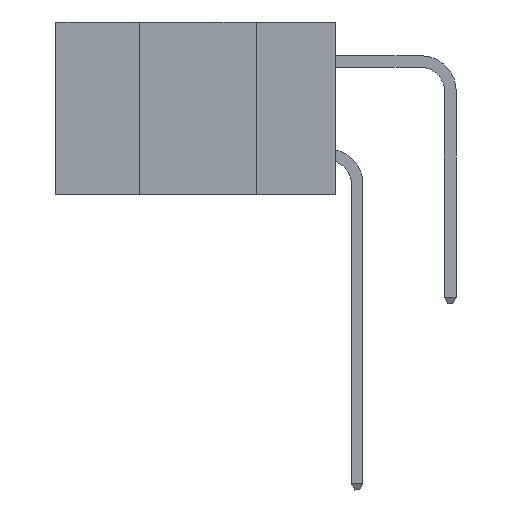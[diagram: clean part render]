
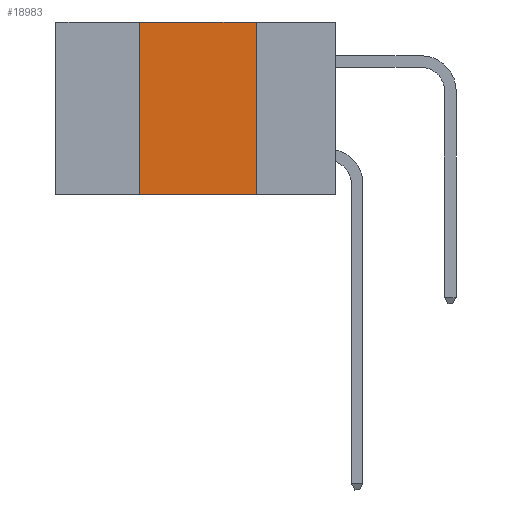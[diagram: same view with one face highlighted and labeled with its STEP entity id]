
A CAD part, left-side view. The second image highlights one B-rep face of the part: STEP entity #18983.
In plain terms, the highlighted planar face has unit normal (-1, 0, 0).
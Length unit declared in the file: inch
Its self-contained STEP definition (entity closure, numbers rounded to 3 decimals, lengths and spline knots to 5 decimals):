
#1022 = EDGE_LOOP ( 'NONE', ( #20843, #13115, #18206, #1481 ) ) ;
#1045 = CARTESIAN_POINT ( 'NONE',  ( 0., 0.42, -0.37 ) ) ;
#1386 = AXIS2_PLACEMENT_3D ( 'NONE', #13677, #13602, #12152 ) ;
#1481 = ORIENTED_EDGE ( 'NONE', *, *, #21602, .T. ) ;
#1672 = LINE ( 'NONE', #15876, #14312 ) ;
#1814 = FACE_OUTER_BOUND ( 'NONE', #1022, .T. ) ;
#1902 = VERTEX_POINT ( 'NONE', #12513 ) ;
#4688 = VECTOR ( 'NONE', #16981, 39.37008 ) ;
#6731 = CARTESIAN_POINT ( 'NONE',  ( 0., 0.17, -0.37 ) ) ;
#6863 = CARTESIAN_POINT ( 'NONE',  ( 0., 0.17, 0. ) ) ;
#7099 = DIRECTION ( 'NONE',  ( 0., -1., 0. ) ) ;
#8546 = PLANE ( 'NONE',  #1386 ) ;
#9239 = LINE ( 'NONE', #13469, #16798 ) ;
#11937 = EDGE_CURVE ( 'NONE', #20999, #1902, #1672, .T. ) ;
#12152 = DIRECTION ( 'NONE',  ( 0., 0., -1. ) ) ;
#12418 = EDGE_CURVE ( 'NONE', #16854, #20999, #12495, .T. ) ;
#12495 = LINE ( 'NONE', #22000, #4688 ) ;
#12513 = CARTESIAN_POINT ( 'NONE',  ( 0., 0.17, 0. ) ) ;
#12937 = EDGE_CURVE ( 'NONE', #1902, #18999, #19840, .T. ) ;
#13115 = ORIENTED_EDGE ( 'NONE', *, *, #11937, .F. ) ;
#13469 = CARTESIAN_POINT ( 'NONE',  ( 0., 0.6, -0.37 ) ) ;
#13602 = DIRECTION ( 'NONE',  ( 1., 0., 0. ) ) ;
#13677 = CARTESIAN_POINT ( 'NONE',  ( 0., 0.6, 0. ) ) ;
#14312 = VECTOR ( 'NONE', #7099, 39.37008 ) ;
#15202 = VECTOR ( 'NONE', #18811, 39.37008 ) ;
#15876 = CARTESIAN_POINT ( 'NONE',  ( 0., 0.6, 0. ) ) ;
#16736 = DIRECTION ( 'NONE',  ( 0., -1., 0. ) ) ;
#16798 = VECTOR ( 'NONE', #16736, 39.37008 ) ;
#16854 = VERTEX_POINT ( 'NONE', #1045 ) ;
#16981 = DIRECTION ( 'NONE',  ( 0., 0., 1. ) ) ;
#18166 = CARTESIAN_POINT ( 'NONE',  ( 0., 0.42, 0. ) ) ;
#18206 = ORIENTED_EDGE ( 'NONE', *, *, #12418, .F. ) ;
#18811 = DIRECTION ( 'NONE',  ( 0., 0., -1. ) ) ;
#18983 = ADVANCED_FACE ( 'NONE', ( #1814 ), #8546, .F. ) ;
#18999 = VERTEX_POINT ( 'NONE', #6731 ) ;
#19840 = LINE ( 'NONE', #6863, #15202 ) ;
#20843 = ORIENTED_EDGE ( 'NONE', *, *, #12937, .F. ) ;
#20999 = VERTEX_POINT ( 'NONE', #18166 ) ;
#21602 = EDGE_CURVE ( 'NONE', #16854, #18999, #9239, .T. ) ;
#22000 = CARTESIAN_POINT ( 'NONE',  ( 0., 0.42, 0. ) ) ;
